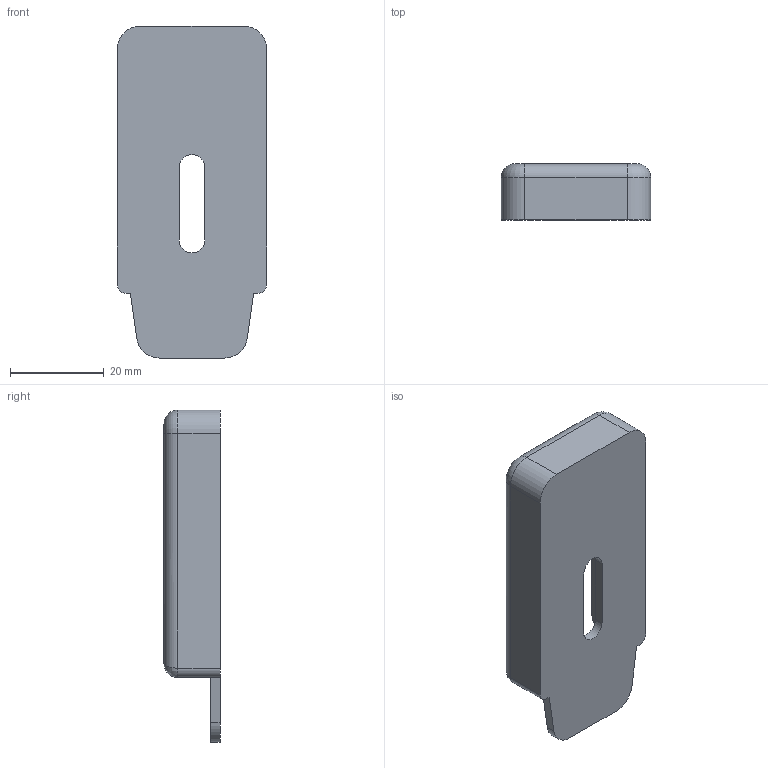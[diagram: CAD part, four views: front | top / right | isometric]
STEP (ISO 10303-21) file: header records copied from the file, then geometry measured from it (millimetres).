
FILE_DESCRIPTION (( 'STEP AP214' ), '1' );
FILE_NAME ('PmagM3Base.STEP', '2020-02-26T02:09:46', ( '' ), ( '' ), 'SwSTEP 2.0', 'SolidWorks 2019', '' );
FILE_SCHEMA (( 'AUTOMOTIVE_DESIGN' ));
Length unit declared in the file: millimetre
Products named in the file (1): PmagM3Base
Bounding box: 32 x 12 x 71 mm (x, y, z)
Volume: 9027 mm3; surface area: 7731.8 mm2
Topology: 1 solids, 1 shells, 65 faces, 169 edges, 104 vertices
Faces by surface type: plane 40, cylinder 21, bspline 2, torus 2
Entity records: 2057 total; most frequent: CARTESIAN_POINT 467, ORIENTED_EDGE 334, DIRECTION 311, EDGE_CURVE 167, LINE 127, VECTOR 127, VERTEX_POINT 104, AXIS2_PLACEMENT_3D 92
